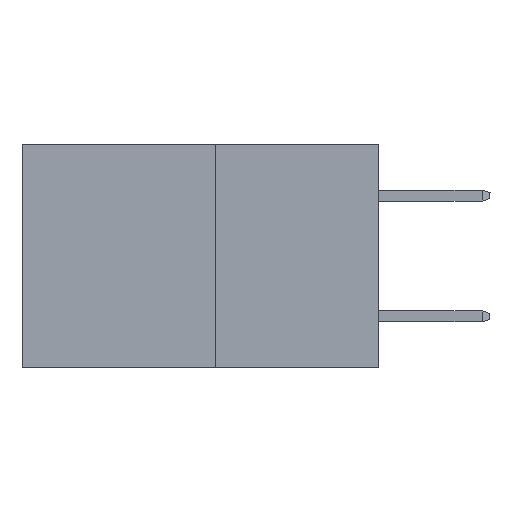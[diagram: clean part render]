
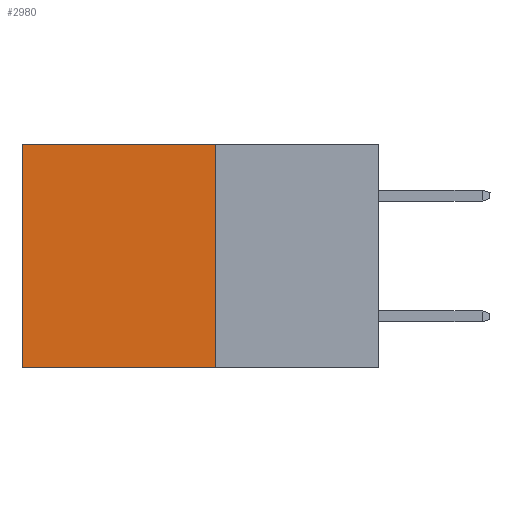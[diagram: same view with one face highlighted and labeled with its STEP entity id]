
A CAD part, left-side view. The second image highlights one B-rep face of the part: STEP entity #2980.
In plain terms, the highlighted planar face has unit normal (-1, 0, 0).
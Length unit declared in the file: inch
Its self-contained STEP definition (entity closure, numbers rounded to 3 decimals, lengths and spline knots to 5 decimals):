
#32 = ORIENTED_EDGE ( 'NONE', *, *, #6044, .T. ) ;
#175 = LINE ( 'NONE', #6382, #8464 ) ;
#424 = VECTOR ( 'NONE', #6812, 39.37008 ) ;
#604 = CARTESIAN_POINT ( 'NONE',  ( 0.277, 0.27, -0.37 ) ) ;
#758 = DIRECTION ( 'NONE',  ( 0., 1., 0. ) ) ;
#897 = VECTOR ( 'NONE', #758, 39.37008 ) ;
#1148 = DIRECTION ( 'NONE',  ( 1., 0., 0. ) ) ;
#1281 = VERTEX_POINT ( 'NONE', #2391 ) ;
#1488 = DIRECTION ( 'NONE',  ( 0., 0., -1. ) ) ;
#1688 = CARTESIAN_POINT ( 'NONE',  ( 0.277, 0.27, 0. ) ) ;
#1881 = PLANE ( 'NONE',  #2696 ) ;
#1991 = CARTESIAN_POINT ( 'NONE',  ( 0.277, 0.59, -0.37 ) ) ;
#2056 = CARTESIAN_POINT ( 'NONE',  ( 0.277, 0.59, -0.37 ) ) ;
#2391 = CARTESIAN_POINT ( 'NONE',  ( 0.277, 0.27, -0.37 ) ) ;
#2503 = EDGE_CURVE ( 'NONE', #9928, #1281, #8824, .T. ) ;
#2696 = AXIS2_PLACEMENT_3D ( 'NONE', #604, #1148, #1488 ) ;
#2980 = ADVANCED_FACE ( 'NONE', ( #7024 ), #1881, .F. ) ;
#3005 = LINE ( 'NONE', #1688, #897 ) ;
#3085 = EDGE_LOOP ( 'NONE', ( #32, #5891, #4053, #3505 ) ) ;
#3190 = DIRECTION ( 'NONE',  ( 0., 0., -1. ) ) ;
#3194 = VERTEX_POINT ( 'NONE', #1991 ) ;
#3312 = VERTEX_POINT ( 'NONE', #5283 ) ;
#3505 = ORIENTED_EDGE ( 'NONE', *, *, #5225, .T. ) ;
#3576 = CARTESIAN_POINT ( 'NONE',  ( 0.277, 0.27, -0.37 ) ) ;
#4053 = ORIENTED_EDGE ( 'NONE', *, *, #2503, .F. ) ;
#4347 = VECTOR ( 'NONE', #3190, 39.37008 ) ;
#4783 = LINE ( 'NONE', #2056, #424 ) ;
#5225 = EDGE_CURVE ( 'NONE', #9928, #3312, #3005, .T. ) ;
#5283 = CARTESIAN_POINT ( 'NONE',  ( 0.277, 0.59, 0. ) ) ;
#5891 = ORIENTED_EDGE ( 'NONE', *, *, #10232, .F. ) ;
#6044 = EDGE_CURVE ( 'NONE', #3312, #3194, #4783, .T. ) ;
#6382 = CARTESIAN_POINT ( 'NONE',  ( 0.277, 0.27, -0.37 ) ) ;
#6418 = DIRECTION ( 'NONE',  ( 0., 1., 0. ) ) ;
#6812 = DIRECTION ( 'NONE',  ( 0., 0., -1. ) ) ;
#7024 = FACE_OUTER_BOUND ( 'NONE', #3085, .T. ) ;
#8434 = CARTESIAN_POINT ( 'NONE',  ( 0.277, 0.27, 0. ) ) ;
#8464 = VECTOR ( 'NONE', #6418, 39.37008 ) ;
#8824 = LINE ( 'NONE', #3576, #4347 ) ;
#9928 = VERTEX_POINT ( 'NONE', #8434 ) ;
#10232 = EDGE_CURVE ( 'NONE', #1281, #3194, #175, .T. ) ;
